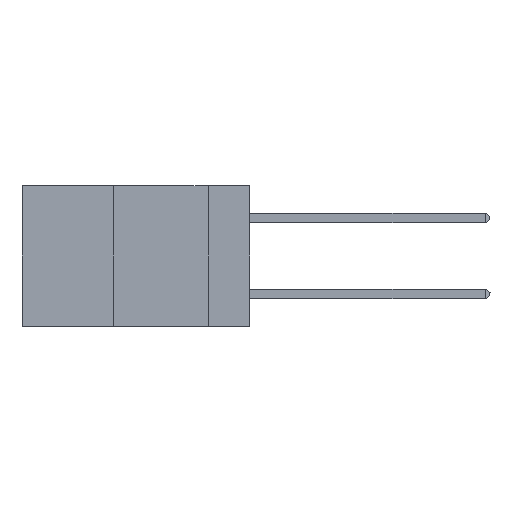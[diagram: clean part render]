
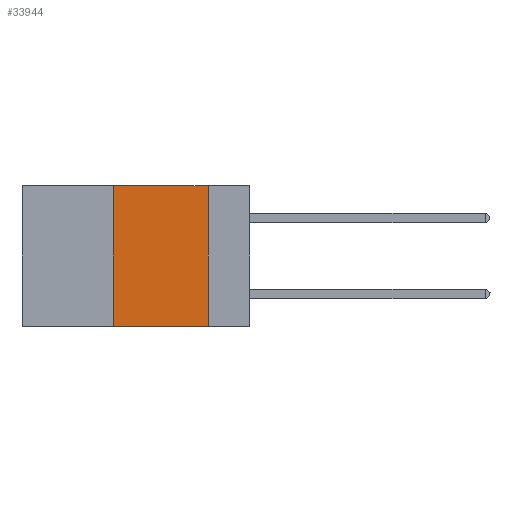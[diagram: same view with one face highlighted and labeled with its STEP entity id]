
A CAD part, left-side view. The second image highlights one B-rep face of the part: STEP entity #33944.
In plain terms, the highlighted planar face has unit normal (-1, 0, 0).
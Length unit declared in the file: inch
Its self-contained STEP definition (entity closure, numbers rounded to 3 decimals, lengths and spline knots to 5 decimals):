
#14 = VECTOR ( 'NONE', #16966, 39.37008 ) ;
#382 = DIRECTION ( 'NONE',  ( 0., 0., -1. ) ) ;
#565 = CARTESIAN_POINT ( 'NONE',  ( 0., 0.6, -0.37 ) ) ;
#5813 = PLANE ( 'NONE',  #33089 ) ;
#6182 = FACE_OUTER_BOUND ( 'NONE', #35474, .T. ) ;
#6297 = CARTESIAN_POINT ( 'NONE',  ( 0., 0.36, -0.37 ) ) ;
#6806 = ORIENTED_EDGE ( 'NONE', *, *, #11046, .F. ) ;
#7332 = VECTOR ( 'NONE', #382, 39.37008 ) ;
#7746 = CARTESIAN_POINT ( 'NONE',  ( 0., 0.36, 0. ) ) ;
#9622 = VERTEX_POINT ( 'NONE', #26332 ) ;
#9710 = VECTOR ( 'NONE', #24796, 39.37008 ) ;
#11046 = EDGE_CURVE ( 'NONE', #21296, #9622, #21934, .T. ) ;
#11327 = CARTESIAN_POINT ( 'NONE',  ( 0., 0.6, 0. ) ) ;
#11599 = VECTOR ( 'NONE', #30938, 39.37008 ) ;
#11668 = DIRECTION ( 'NONE',  ( 1., 0., 0. ) ) ;
#11854 = DIRECTION ( 'NONE',  ( 0., 0., -1. ) ) ;
#13822 = LINE ( 'NONE', #24993, #9710 ) ;
#15280 = ORIENTED_EDGE ( 'NONE', *, *, #18233, .F. ) ;
#16966 = DIRECTION ( 'NONE',  ( 0., -1., 0. ) ) ;
#17337 = CARTESIAN_POINT ( 'NONE',  ( 0., 0.6, 0. ) ) ;
#17903 = LINE ( 'NONE', #25619, #7332 ) ;
#18233 = EDGE_CURVE ( 'NONE', #9622, #33763, #17903, .T. ) ;
#19120 = EDGE_CURVE ( 'NONE', #33532, #21296, #13822, .T. ) ;
#21296 = VERTEX_POINT ( 'NONE', #7746 ) ;
#21553 = CARTESIAN_POINT ( 'NONE',  ( 0., 0.11, -0.37 ) ) ;
#21934 = LINE ( 'NONE', #11327, #14 ) ;
#22517 = LINE ( 'NONE', #565, #11599 ) ;
#24796 = DIRECTION ( 'NONE',  ( 0., 0., 1. ) ) ;
#24993 = CARTESIAN_POINT ( 'NONE',  ( 0., 0.36, 0. ) ) ;
#25619 = CARTESIAN_POINT ( 'NONE',  ( 0., 0.11, 0. ) ) ;
#26332 = CARTESIAN_POINT ( 'NONE',  ( 0., 0.11, 0. ) ) ;
#30938 = DIRECTION ( 'NONE',  ( 0., -1., 0. ) ) ;
#33089 = AXIS2_PLACEMENT_3D ( 'NONE', #17337, #11668, #11854 ) ;
#33532 = VERTEX_POINT ( 'NONE', #6297 ) ;
#33763 = VERTEX_POINT ( 'NONE', #21553 ) ;
#33944 = ADVANCED_FACE ( 'NONE', ( #6182 ), #5813, .F. ) ;
#34286 = ORIENTED_EDGE ( 'NONE', *, *, #34801, .T. ) ;
#34773 = ORIENTED_EDGE ( 'NONE', *, *, #19120, .F. ) ;
#34801 = EDGE_CURVE ( 'NONE', #33532, #33763, #22517, .T. ) ;
#35474 = EDGE_LOOP ( 'NONE', ( #15280, #6806, #34773, #34286 ) ) ;
